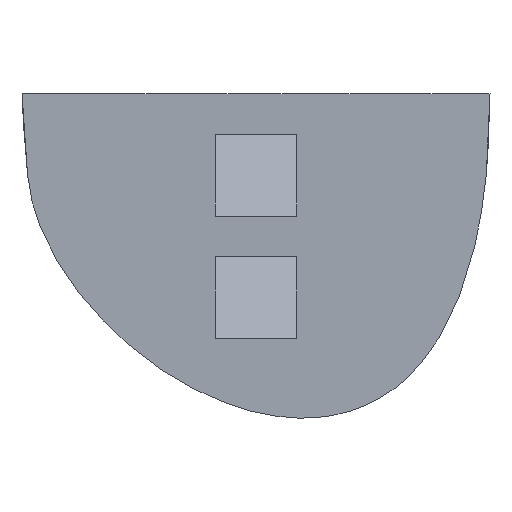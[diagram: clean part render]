
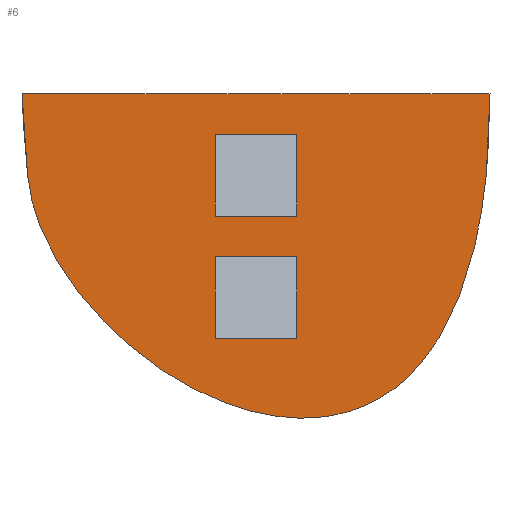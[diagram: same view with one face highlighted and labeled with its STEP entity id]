
A CAD part, left-side view. The second image highlights one B-rep face of the part: STEP entity #6.
In plain terms, the highlighted planar face has unit normal (-1, 0, 0).
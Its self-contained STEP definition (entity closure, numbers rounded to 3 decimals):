
#5 = EDGE_LOOP ( 'NONE', ( #218, #143, #125, #229 ) ) ;
#6 = ADVANCED_FACE ( 'NONE', ( #339, #394, #122 ), #433, .T. ) ;
#7 = CARTESIAN_POINT ( 'NONE',  ( -10., -14.361, 0. ) ) ;
#8 = CARTESIAN_POINT ( 'NONE',  ( -10., 14.361, 0. ) ) ;
#10 = CARTESIAN_POINT ( 'NONE',  ( -10., 14.361, -0.535 ) ) ;
#11 = CARTESIAN_POINT ( 'NONE',  ( -10., 14.326, -1.374 ) ) ;
#13 = CARTESIAN_POINT ( 'NONE',  ( -10., 14.244, -2.502 ) ) ;
#15 = CARTESIAN_POINT ( 'NONE',  ( -10., 14.14, -3.634 ) ) ;
#16 = DIRECTION ( 'NONE',  ( 0., 0., 1. ) ) ;
#24 = LINE ( 'NONE', #445, #121 ) ;
#33 = CARTESIAN_POINT ( 'NONE',  ( -10., 14.061, -4.467 ) ) ;
#34 = VERTEX_POINT ( 'NONE', #397 ) ;
#35 = CARTESIAN_POINT ( 'NONE',  ( -10., 14.017, -5. ) ) ;
#37 = VECTOR ( 'NONE', #86, 1000. ) ;
#39 = CARTESIAN_POINT ( 'NONE',  ( -10., 14.017, -5. ) ) ;
#40 = CARTESIAN_POINT ( 'NONE',  ( -10., 2.5, -2.5 ) ) ;
#41 = VECTOR ( 'NONE', #59, 1000. ) ;
#42 = VECTOR ( 'NONE', #84, 1000. ) ;
#44 = B_SPLINE_CURVE_WITH_KNOTS ( 'NONE', 3,
 ( #39, #58, #35, #33, #15, #13, #11, #10, #8 ),
 .UNSPECIFIED., .F., .F.,
 ( 4, 2, 1, 1, 1, 4 ),
 ( 0., 0., 0.25, 0.5, 0.75, 1. ),
 .UNSPECIFIED. ) ;
#47 = VERTEX_POINT ( 'NONE', #395 ) ;
#56 = DIRECTION ( 'NONE',  ( 0., 0., 1. ) ) ;
#58 = CARTESIAN_POINT ( 'NONE',  ( -10., 14.017, -5. ) ) ;
#59 = DIRECTION ( 'NONE',  ( 0., -1., 0. ) ) ;
#60 = CARTESIAN_POINT ( 'NONE',  ( -10., -14.361, -1.01 ) ) ;
#61 = CARTESIAN_POINT ( 'NONE',  ( -10., 7.908, -15.41 ) ) ;
#65 = CARTESIAN_POINT ( 'NONE',  ( -10., 2.5, -2.5 ) ) ;
#66 = VERTEX_POINT ( 'NONE', #385 ) ;
#69 = CARTESIAN_POINT ( 'NONE',  ( -10., 14.361, 0. ) ) ;
#70 = VERTEX_POINT ( 'NONE', #347 ) ;
#72 = CARTESIAN_POINT ( 'NONE',  ( -10., -12.669, -12.171 ) ) ;
#73 = CARTESIAN_POINT ( 'NONE',  ( -10., 5.385, -17.288 ) ) ;
#83 = ORIENTED_EDGE ( 'NONE', *, *, #292, .F. ) ;
#84 = DIRECTION ( 'NONE',  ( 0., -1., 0. ) ) ;
#86 = DIRECTION ( 'NONE',  ( 0., -1., 0. ) ) ;
#88 = LINE ( 'NONE', #128, #266 ) ;
#91 = CARTESIAN_POINT ( 'NONE',  ( -10., 2.5, -7.5 ) ) ;
#92 = CARTESIAN_POINT ( 'NONE',  ( -10., 2.5, -2.5 ) ) ;
#93 = CARTESIAN_POINT ( 'NONE',  ( -10., 12.012, -10.737 ) ) ;
#95 = LINE ( 'NONE', #443, #447 ) ;
#96 = ORIENTED_EDGE ( 'NONE', *, *, #359, .T. ) ;
#101 = DIRECTION ( 'NONE',  ( 0., -1., 0. ) ) ;
#115 = B_SPLINE_CURVE_WITH_KNOTS ( 'NONE', 3,
 ( #7, #60, #175, #405, #283, #72, #403, #267, #303, #179, #322, #361, #73, #61, #349, #93, #132, #308, #392 ),
 .UNSPECIFIED., .F., .F.,
 ( 4, 1, 1, 1, 1, 1, 1, 1, 1, 1, 1, 1, 1, 1, 1, 1, 4 ),
 ( 0., 0.063, 0.125, 0.188, 0.25, 0.313, 0.375, 0.438, 0.5, 0.563, 0.625, 0.688, 0.75, 0.813, 0.875, 0.938, 1. ),
 .UNSPECIFIED. ) ;
#120 = DIRECTION ( 'NONE',  ( 0., 0., 1. ) ) ;
#121 = VECTOR ( 'NONE', #139, 1000. ) ;
#122 = FACE_BOUND ( 'NONE', #5, .T. ) ;
#125 = ORIENTED_EDGE ( 'NONE', *, *, #260, .F. ) ;
#126 = CARTESIAN_POINT ( 'NONE',  ( -10., 2.5, -7.5 ) ) ;
#128 = CARTESIAN_POINT ( 'NONE',  ( -10., -2.5, -2.5 ) ) ;
#131 = ORIENTED_EDGE ( 'NONE', *, *, #259, .F. ) ;
#132 = CARTESIAN_POINT ( 'NONE',  ( -10., 13.43, -7.995 ) ) ;
#133 = CARTESIAN_POINT ( 'NONE',  ( -10., -2.5, -10. ) ) ;
#134 = CARTESIAN_POINT ( 'NONE',  ( -10., 2.5, -15. ) ) ;
#139 = DIRECTION ( 'NONE',  ( 0., 0., 1. ) ) ;
#141 = VERTEX_POINT ( 'NONE', #301 ) ;
#143 = ORIENTED_EDGE ( 'NONE', *, *, #248, .F. ) ;
#153 = ORIENTED_EDGE ( 'NONE', *, *, #387, .F. ) ;
#164 = VERTEX_POINT ( 'NONE', #241 ) ;
#175 = CARTESIAN_POINT ( 'NONE',  ( -10., -14.311, -3.041 ) ) ;
#178 = ORIENTED_EDGE ( 'NONE', *, *, #325, .F. ) ;
#179 = CARTESIAN_POINT ( 'NONE',  ( -10., -3.599, -20.045 ) ) ;
#198 = ORIENTED_EDGE ( 'NONE', *, *, #296, .F. ) ;
#204 = VECTOR ( 'NONE', #56, 1000. ) ;
#208 = VERTEX_POINT ( 'NONE', #210 ) ;
#210 = CARTESIAN_POINT ( 'NONE',  ( -10., 14.017, -5. ) ) ;
#218 = ORIENTED_EDGE ( 'NONE', *, *, #279, .T. ) ;
#229 = ORIENTED_EDGE ( 'NONE', *, *, #281, .T. ) ;
#240 = VERTEX_POINT ( 'NONE', #126 ) ;
#241 = CARTESIAN_POINT ( 'NONE',  ( -10., 2.5, -10. ) ) ;
#248 = EDGE_CURVE ( 'NONE', #402, #66, #88, .T. ) ;
#259 = EDGE_CURVE ( 'NONE', #47, #34, #297, .T. ) ;
#260 = EDGE_CURVE ( 'NONE', #240, #402, #324, .T. ) ;
#266 = VECTOR ( 'NONE', #120, 1000. ) ;
#267 = CARTESIAN_POINT ( 'NONE',  ( -10., -9.401, -17.545 ) ) ;
#279 = EDGE_CURVE ( 'NONE', #333, #66, #302, .T. ) ;
#280 = CARTESIAN_POINT ( 'NONE',  ( -10., -2.5, -7.5 ) ) ;
#281 = EDGE_CURVE ( 'NONE', #240, #333, #353, .T. ) ;
#283 = CARTESIAN_POINT ( 'NONE',  ( -10., -13.526, -9.164 ) ) ;
#292 = EDGE_CURVE ( 'NONE', #208, #432, #44, .T. ) ;
#296 = EDGE_CURVE ( 'NONE', #70, #208, #115, .T. ) ;
#297 = LINE ( 'NONE', #134, #37 ) ;
#301 = CARTESIAN_POINT ( 'NONE',  ( -10., -2.5, -10. ) ) ;
#302 = LINE ( 'NONE', #92, #41 ) ;
#303 = CARTESIAN_POINT ( 'NONE',  ( -10., -6.733, -19.335 ) ) ;
#308 = CARTESIAN_POINT ( 'NONE',  ( -10., 13.933, -6.007 ) ) ;
#318 = EDGE_LOOP ( 'NONE', ( #401, #178, #131, #96 ) ) ;
#319 = DIRECTION ( 'NONE',  ( 0., -1., 0. ) ) ;
#322 = CARTESIAN_POINT ( 'NONE',  ( -10., -0.419, -19.767 ) ) ;
#324 = LINE ( 'NONE', #91, #42 ) ;
#325 = EDGE_CURVE ( 'NONE', #34, #141, #415, .T. ) ;
#333 = VERTEX_POINT ( 'NONE', #40 ) ;
#339 = FACE_BOUND ( 'NONE', #318, .T. ) ;
#347 = CARTESIAN_POINT ( 'NONE',  ( -10., -14.361, 0. ) ) ;
#349 = CARTESIAN_POINT ( 'NONE',  ( -10., 10.136, -13.215 ) ) ;
#353 = LINE ( 'NONE', #65, #204 ) ;
#359 = EDGE_CURVE ( 'NONE', #47, #164, #24, .T. ) ;
#361 = CARTESIAN_POINT ( 'NONE',  ( -10., 2.599, -18.781 ) ) ;
#380 = EDGE_LOOP ( 'NONE', ( #198, #153, #83 ) ) ;
#385 = CARTESIAN_POINT ( 'NONE',  ( -10., -2.5, -2.5 ) ) ;
#387 = EDGE_CURVE ( 'NONE', #432, #70, #95, .T. ) ;
#392 = CARTESIAN_POINT ( 'NONE',  ( -10., 14.017, -5. ) ) ;
#393 = VECTOR ( 'NONE', #16, 1000. ) ;
#394 = FACE_OUTER_BOUND ( 'NONE', #380, .T. ) ;
#395 = CARTESIAN_POINT ( 'NONE',  ( -10., 2.5, -15. ) ) ;
#397 = CARTESIAN_POINT ( 'NONE',  ( -10., -2.5, -15. ) ) ;
#401 = ORIENTED_EDGE ( 'NONE', *, *, #417, .T. ) ;
#402 = VERTEX_POINT ( 'NONE', #280 ) ;
#403 = CARTESIAN_POINT ( 'NONE',  ( -10., -11.347, -15.03 ) ) ;
#404 = CARTESIAN_POINT ( 'NONE',  ( -10., 2.5, -10. ) ) ;
#405 = CARTESIAN_POINT ( 'NONE',  ( -10., -14.045, -6.105 ) ) ;
#415 = LINE ( 'NONE', #133, #393 ) ;
#417 = EDGE_CURVE ( 'NONE', #164, #141, #446, .T. ) ;
#422 = CARTESIAN_POINT ( 'NONE',  ( -10., -0.559, -19.672 ) ) ;
#424 = DIRECTION ( 'NONE',  ( -1., 0., 0. ) ) ;
#432 = VERTEX_POINT ( 'NONE', #69 ) ;
#433 = PLANE ( 'NONE',  #464 ) ;
#436 = DIRECTION ( 'NONE',  ( 0., 0., -1. ) ) ;
#443 = CARTESIAN_POINT ( 'NONE',  ( -10., -14.361, 0. ) ) ;
#445 = CARTESIAN_POINT ( 'NONE',  ( -10., 2.5, -10. ) ) ;
#446 = LINE ( 'NONE', #404, #448 ) ;
#447 = VECTOR ( 'NONE', #319, 1000. ) ;
#448 = VECTOR ( 'NONE', #101, 1000. ) ;
#464 = AXIS2_PLACEMENT_3D ( 'NONE', #422, #424, #436 ) ;
